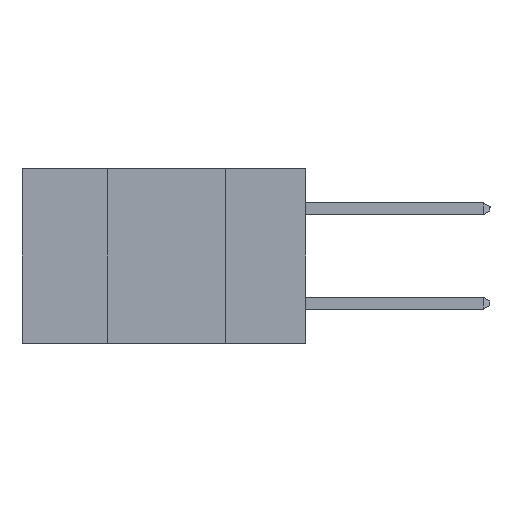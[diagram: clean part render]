
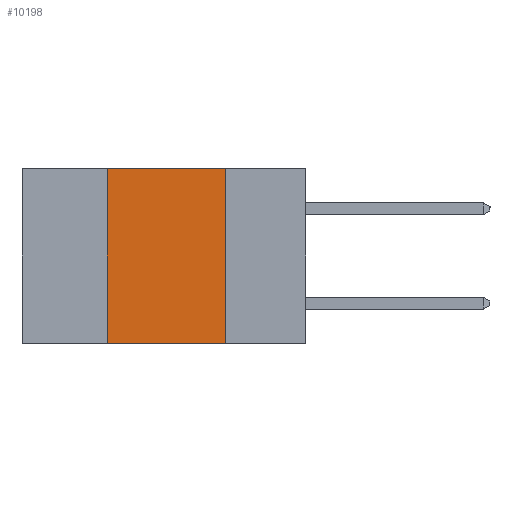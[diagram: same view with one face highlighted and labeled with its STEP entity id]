
A CAD part, left-side view. The second image highlights one B-rep face of the part: STEP entity #10198.
In plain terms, the highlighted planar face has unit normal (-1, 0, 0).
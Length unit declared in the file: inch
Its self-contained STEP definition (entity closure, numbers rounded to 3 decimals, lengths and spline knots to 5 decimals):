
#612 = LINE ( 'NONE', #8406, #6130 ) ;
#889 = VERTEX_POINT ( 'NONE', #5038 ) ;
#1242 = EDGE_CURVE ( 'NONE', #3852, #889, #612, .T. ) ;
#1381 = VECTOR ( 'NONE', #1723, 39.37008 ) ;
#1723 = DIRECTION ( 'NONE',  ( 0., -1., 0. ) ) ;
#2136 = ORIENTED_EDGE ( 'NONE', *, *, #9896, .T. ) ;
#2183 = DIRECTION ( 'NONE',  ( 1., 0., 0. ) ) ;
#2292 = CARTESIAN_POINT ( 'NONE',  ( 0., 0.17, 0. ) ) ;
#2382 = EDGE_CURVE ( 'NONE', #9861, #13761, #8097, .T. ) ;
#2751 = CARTESIAN_POINT ( 'NONE',  ( 0., 0.17, -0.37 ) ) ;
#3034 = LINE ( 'NONE', #13317, #1381 ) ;
#3387 = PLANE ( 'NONE',  #6495 ) ;
#3852 = VERTEX_POINT ( 'NONE', #11231 ) ;
#4272 = EDGE_CURVE ( 'NONE', #889, #9861, #3034, .T. ) ;
#4385 = ORIENTED_EDGE ( 'NONE', *, *, #2382, .F. ) ;
#5038 = CARTESIAN_POINT ( 'NONE',  ( 0., 0.42, 0. ) ) ;
#5722 = CARTESIAN_POINT ( 'NONE',  ( 0., 0.6, -0.37 ) ) ;
#6130 = VECTOR ( 'NONE', #16076, 39.37008 ) ;
#6495 = AXIS2_PLACEMENT_3D ( 'NONE', #8675, #2183, #13959 ) ;
#8097 = LINE ( 'NONE', #2751, #14455 ) ;
#8229 = LINE ( 'NONE', #5722, #12595 ) ;
#8406 = CARTESIAN_POINT ( 'NONE',  ( 0., 0.42, -0.37 ) ) ;
#8675 = CARTESIAN_POINT ( 'NONE',  ( 0., 0.6, 0. ) ) ;
#9025 = CARTESIAN_POINT ( 'NONE',  ( 0., 0.17, -0.37 ) ) ;
#9121 = ORIENTED_EDGE ( 'NONE', *, *, #1242, .F. ) ;
#9489 = DIRECTION ( 'NONE',  ( 0., 0., -1. ) ) ;
#9803 = FACE_OUTER_BOUND ( 'NONE', #16368, .T. ) ;
#9861 = VERTEX_POINT ( 'NONE', #2292 ) ;
#9896 = EDGE_CURVE ( 'NONE', #3852, #13761, #8229, .T. ) ;
#10198 = ADVANCED_FACE ( 'NONE', ( #9803 ), #3387, .F. ) ;
#11231 = CARTESIAN_POINT ( 'NONE',  ( 0., 0.42, -0.37 ) ) ;
#12595 = VECTOR ( 'NONE', #16003, 39.37008 ) ;
#13317 = CARTESIAN_POINT ( 'NONE',  ( 0., 0.6, 0. ) ) ;
#13761 = VERTEX_POINT ( 'NONE', #9025 ) ;
#13959 = DIRECTION ( 'NONE',  ( 0., 0., -1. ) ) ;
#14455 = VECTOR ( 'NONE', #9489, 39.37008 ) ;
#16003 = DIRECTION ( 'NONE',  ( 0., -1., 0. ) ) ;
#16076 = DIRECTION ( 'NONE',  ( 0., 0., 1. ) ) ;
#16368 = EDGE_LOOP ( 'NONE', ( #4385, #16536, #9121, #2136 ) ) ;
#16536 = ORIENTED_EDGE ( 'NONE', *, *, #4272, .F. ) ;
